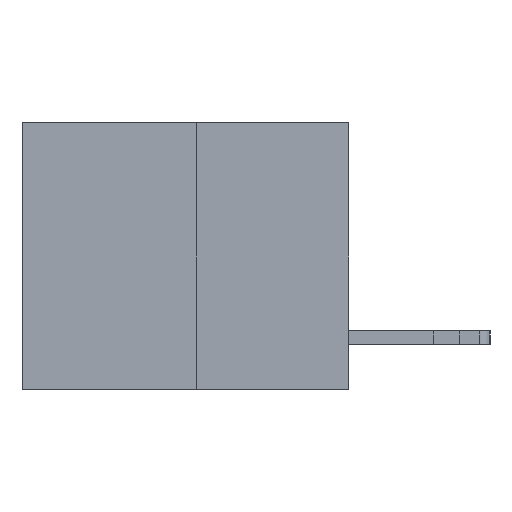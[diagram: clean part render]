
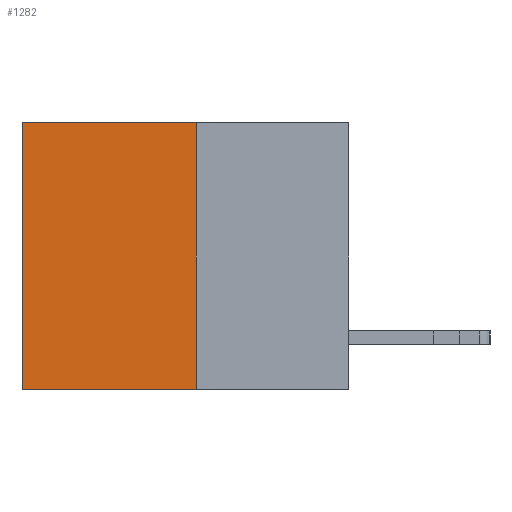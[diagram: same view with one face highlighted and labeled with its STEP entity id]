
A CAD part, left-side view. The second image highlights one B-rep face of the part: STEP entity #1282.
In plain terms, the highlighted planar face has unit normal (-1, 0, 0).
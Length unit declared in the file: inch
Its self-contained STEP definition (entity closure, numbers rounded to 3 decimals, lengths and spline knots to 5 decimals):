
#2 = VERTEX_POINT ( 'NONE', #11522 ) ;
#1167 = LINE ( 'NONE', #12896, #17521 ) ;
#1282 = ADVANCED_FACE ( 'NONE', ( #17071 ), #1940, .F. ) ;
#1940 = PLANE ( 'NONE',  #8657 ) ;
#2155 = CARTESIAN_POINT ( 'NONE',  ( 0.3165, 0.6, -0.49 ) ) ;
#3138 = EDGE_CURVE ( 'NONE', #2, #12576, #7345, .T. ) ;
#4777 = EDGE_CURVE ( 'NONE', #2, #9656, #18740, .T. ) ;
#5556 = CARTESIAN_POINT ( 'NONE',  ( 0.3165, 0.28, 0. ) ) ;
#5962 = DIRECTION ( 'NONE',  ( 0., 0., -1. ) ) ;
#6548 = CARTESIAN_POINT ( 'NONE',  ( 0.3165, 0.28, -0.49 ) ) ;
#6634 = DIRECTION ( 'NONE',  ( 0., 0., -1. ) ) ;
#7345 = LINE ( 'NONE', #6548, #14054 ) ;
#8649 = VECTOR ( 'NONE', #12873, 39.37008 ) ;
#8657 = AXIS2_PLACEMENT_3D ( 'NONE', #16278, #26447, #5962 ) ;
#9656 = VERTEX_POINT ( 'NONE', #18931 ) ;
#11178 = DIRECTION ( 'NONE',  ( 0., 1., 0. ) ) ;
#11522 = CARTESIAN_POINT ( 'NONE',  ( 0.3165, 0.28, 0. ) ) ;
#11787 = ORIENTED_EDGE ( 'NONE', *, *, #4777, .T. ) ;
#12576 = VERTEX_POINT ( 'NONE', #25446 ) ;
#12873 = DIRECTION ( 'NONE',  ( 0., 0., -1. ) ) ;
#12896 = CARTESIAN_POINT ( 'NONE',  ( 0.3165, 0.28, -0.49 ) ) ;
#14054 = VECTOR ( 'NONE', #6634, 39.37008 ) ;
#14169 = VERTEX_POINT ( 'NONE', #2155 ) ;
#14247 = ORIENTED_EDGE ( 'NONE', *, *, #3138, .F. ) ;
#16278 = CARTESIAN_POINT ( 'NONE',  ( 0.3165, 0.28, -0.49 ) ) ;
#17071 = FACE_OUTER_BOUND ( 'NONE', #18320, .T. ) ;
#17475 = ORIENTED_EDGE ( 'NONE', *, *, #22141, .F. ) ;
#17521 = VECTOR ( 'NONE', #11178, 39.37008 ) ;
#17630 = LINE ( 'NONE', #25256, #8649 ) ;
#18320 = EDGE_LOOP ( 'NONE', ( #25624, #17475, #14247, #11787 ) ) ;
#18740 = LINE ( 'NONE', #5556, #20377 ) ;
#18931 = CARTESIAN_POINT ( 'NONE',  ( 0.3165, 0.6, 0. ) ) ;
#19804 = DIRECTION ( 'NONE',  ( 0., 1., 0. ) ) ;
#20377 = VECTOR ( 'NONE', #19804, 39.37008 ) ;
#22141 = EDGE_CURVE ( 'NONE', #12576, #14169, #1167, .T. ) ;
#24864 = EDGE_CURVE ( 'NONE', #9656, #14169, #17630, .T. ) ;
#25256 = CARTESIAN_POINT ( 'NONE',  ( 0.3165, 0.6, -0.49 ) ) ;
#25446 = CARTESIAN_POINT ( 'NONE',  ( 0.3165, 0.28, -0.49 ) ) ;
#25624 = ORIENTED_EDGE ( 'NONE', *, *, #24864, .T. ) ;
#26447 = DIRECTION ( 'NONE',  ( 1., 0., 0. ) ) ;
